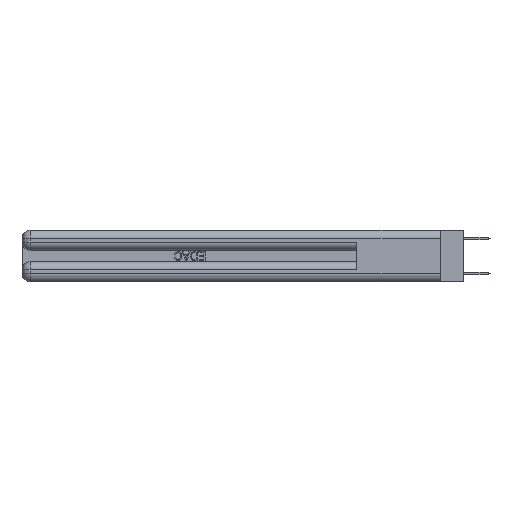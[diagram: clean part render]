
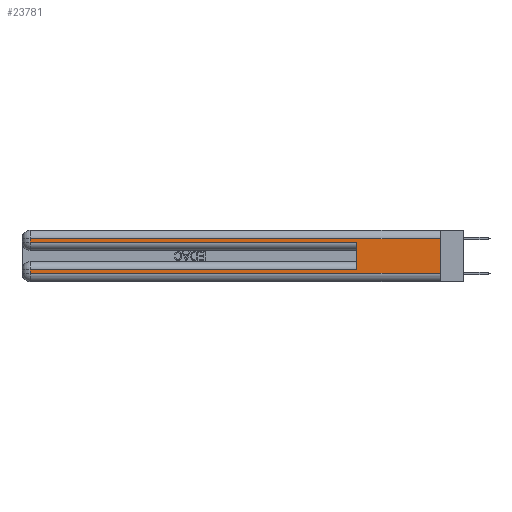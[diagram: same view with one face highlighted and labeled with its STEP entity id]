
A CAD part, left-side view. The second image highlights one B-rep face of the part: STEP entity #23781.
In plain terms, the highlighted planar face has unit normal (-1, 0, 0).
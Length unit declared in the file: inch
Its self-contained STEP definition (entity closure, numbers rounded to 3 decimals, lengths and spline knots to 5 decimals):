
#919 = ORIENTED_EDGE ( 'NONE', *, *, #18726, .T. ) ;
#1191 = EDGE_CURVE ( 'NONE', #10408, #19852, #8428, .T. ) ;
#1807 = DIRECTION ( 'NONE',  ( 0., -1., 0. ) ) ;
#2237 = DIRECTION ( 'NONE',  ( 1., 0., 0. ) ) ;
#2418 = VECTOR ( 'NONE', #15590, 39.37008 ) ;
#2734 = EDGE_CURVE ( 'NONE', #21792, #30571, #17704, .T. ) ;
#3184 = ORIENTED_EDGE ( 'NONE', *, *, #33218, .T. ) ;
#3833 = CARTESIAN_POINT ( 'NONE',  ( 0., 2.94, 0.37 ) ) ;
#3862 = DIRECTION ( 'NONE',  ( 0., 1., 0. ) ) ;
#3983 = VECTOR ( 'NONE', #9393, 39.37008 ) ;
#4085 = EDGE_CURVE ( 'NONE', #10408, #7689, #7096, .T. ) ;
#4196 = EDGE_CURVE ( 'NONE', #11440, #19445, #20891, .T. ) ;
#4791 = EDGE_CURVE ( 'NONE', #19445, #7689, #16450, .T. ) ;
#4830 = CARTESIAN_POINT ( 'NONE',  ( 0., 0., 0.06 ) ) ;
#7096 = LINE ( 'NONE', #24797, #30934 ) ;
#7421 = AXIS2_PLACEMENT_3D ( 'NONE', #8128, #2237, #18078 ) ;
#7689 = VERTEX_POINT ( 'NONE', #30127 ) ;
#7794 = PLANE ( 'NONE',  #7421 ) ;
#8128 = CARTESIAN_POINT ( 'NONE',  ( 0., 0., 0.37 ) ) ;
#8428 = LINE ( 'NONE', #29162, #14371 ) ;
#8749 = EDGE_CURVE ( 'NONE', #21709, #30571, #25233, .T. ) ;
#8999 = ORIENTED_EDGE ( 'NONE', *, *, #8749, .T. ) ;
#9034 = CARTESIAN_POINT ( 'NONE',  ( 0., 2.94, 0.085 ) ) ;
#9393 = DIRECTION ( 'NONE',  ( 0., 0., -1. ) ) ;
#9650 = ORIENTED_EDGE ( 'NONE', *, *, #4085, .F. ) ;
#9939 = VECTOR ( 'NONE', #15180, 39.37008 ) ;
#10288 = DIRECTION ( 'NONE',  ( 0., 0., -1. ) ) ;
#10408 = VERTEX_POINT ( 'NONE', #24219 ) ;
#11440 = VERTEX_POINT ( 'NONE', #11968 ) ;
#11968 = CARTESIAN_POINT ( 'NONE',  ( 0., 2.94, 0.31 ) ) ;
#12055 = VECTOR ( 'NONE', #10288, 39.37008 ) ;
#12279 = VECTOR ( 'NONE', #1807, 39.37008 ) ;
#12468 = CARTESIAN_POINT ( 'NONE',  ( 0., 0., 0.37 ) ) ;
#13673 = CARTESIAN_POINT ( 'NONE',  ( 0., 0., 0.31 ) ) ;
#13757 = CARTESIAN_POINT ( 'NONE',  ( 0., 0., 0.285 ) ) ;
#14371 = VECTOR ( 'NONE', #3862, 39.37008 ) ;
#14843 = ORIENTED_EDGE ( 'NONE', *, *, #2734, .F. ) ;
#14971 = CARTESIAN_POINT ( 'NONE',  ( 0., 2.94, 0.285 ) ) ;
#15180 = DIRECTION ( 'NONE',  ( 0., 0., -1. ) ) ;
#15590 = DIRECTION ( 'NONE',  ( 0., 1., 0. ) ) ;
#15993 = EDGE_LOOP ( 'NONE', ( #14843, #919, #27480, #20578, #9650, #32825, #3184, #8999 ) ) ;
#16450 = LINE ( 'NONE', #13757, #18592 ) ;
#17704 = LINE ( 'NONE', #12468, #12055 ) ;
#18006 = CARTESIAN_POINT ( 'NONE',  ( 0., 0., 0.06 ) ) ;
#18078 = DIRECTION ( 'NONE',  ( 0., 0., -1. ) ) ;
#18211 = CARTESIAN_POINT ( 'NONE',  ( 0., 2.94, 0.37 ) ) ;
#18592 = VECTOR ( 'NONE', #31307, 39.37008 ) ;
#18726 = EDGE_CURVE ( 'NONE', #21792, #11440, #20957, .T. ) ;
#19445 = VERTEX_POINT ( 'NONE', #14971 ) ;
#19852 = VERTEX_POINT ( 'NONE', #9034 ) ;
#20578 = ORIENTED_EDGE ( 'NONE', *, *, #4791, .T. ) ;
#20891 = LINE ( 'NONE', #18211, #9939 ) ;
#20957 = LINE ( 'NONE', #28726, #2418 ) ;
#21709 = VERTEX_POINT ( 'NONE', #23633 ) ;
#21792 = VERTEX_POINT ( 'NONE', #13673 ) ;
#23633 = CARTESIAN_POINT ( 'NONE',  ( 0., 2.94, 0.06 ) ) ;
#23781 = ADVANCED_FACE ( 'NONE', ( #31231 ), #7794, .F. ) ;
#24219 = CARTESIAN_POINT ( 'NONE',  ( 0., 0.6, 0.085 ) ) ;
#24797 = CARTESIAN_POINT ( 'NONE',  ( 0., 0.6, 0.145 ) ) ;
#25233 = LINE ( 'NONE', #4830, #12279 ) ;
#27480 = ORIENTED_EDGE ( 'NONE', *, *, #4196, .T. ) ;
#27496 = DIRECTION ( 'NONE',  ( 0., 0., 1. ) ) ;
#28726 = CARTESIAN_POINT ( 'NONE',  ( 0., 0., 0.31 ) ) ;
#29162 = CARTESIAN_POINT ( 'NONE',  ( 0., 0., 0.085 ) ) ;
#29632 = LINE ( 'NONE', #3833, #3983 ) ;
#30127 = CARTESIAN_POINT ( 'NONE',  ( 0., 0.6, 0.285 ) ) ;
#30571 = VERTEX_POINT ( 'NONE', #18006 ) ;
#30934 = VECTOR ( 'NONE', #27496, 39.37008 ) ;
#31231 = FACE_OUTER_BOUND ( 'NONE', #15993, .T. ) ;
#31307 = DIRECTION ( 'NONE',  ( 0., -1., 0. ) ) ;
#32825 = ORIENTED_EDGE ( 'NONE', *, *, #1191, .T. ) ;
#33218 = EDGE_CURVE ( 'NONE', #19852, #21709, #29632, .T. ) ;
